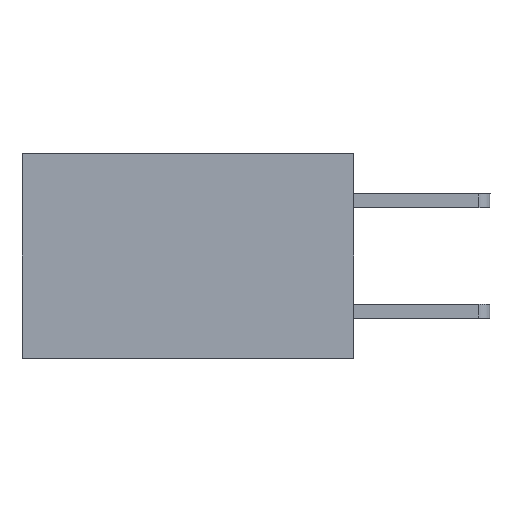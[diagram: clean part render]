
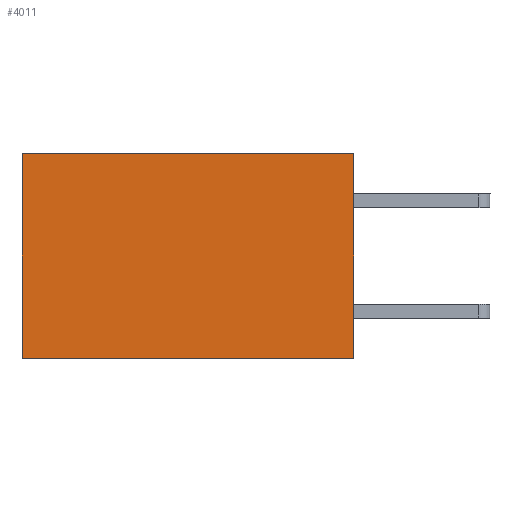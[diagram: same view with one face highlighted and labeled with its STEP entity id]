
A CAD part, left-side view. The second image highlights one B-rep face of the part: STEP entity #4011.
In plain terms, the highlighted planar face has unit normal (-1, 0, 0).
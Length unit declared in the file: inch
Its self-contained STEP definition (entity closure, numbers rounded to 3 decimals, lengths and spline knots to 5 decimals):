
#137 = VERTEX_POINT ( 'NONE', #3041 ) ;
#629 = VERTEX_POINT ( 'NONE', #8967 ) ;
#1329 = CARTESIAN_POINT ( 'NONE',  ( 0.2875, 0., -0.37 ) ) ;
#1948 = DIRECTION ( 'NONE',  ( 0., 0., -1. ) ) ;
#2176 = VECTOR ( 'NONE', #7032, 39.37008 ) ;
#2194 = ORIENTED_EDGE ( 'NONE', *, *, #3155, .T. ) ;
#2203 = CARTESIAN_POINT ( 'NONE',  ( 0.2875, 0., 0. ) ) ;
#2215 = EDGE_CURVE ( 'NONE', #8584, #6229, #4399, .T. ) ;
#2803 = LINE ( 'NONE', #6075, #2176 ) ;
#3041 = CARTESIAN_POINT ( 'NONE',  ( 0.2875, 0.6, -0.37 ) ) ;
#3075 = LINE ( 'NONE', #1329, #7894 ) ;
#3109 = VECTOR ( 'NONE', #10607, 39.37008 ) ;
#3155 = EDGE_CURVE ( 'NONE', #629, #137, #8492, .T. ) ;
#3424 = FACE_OUTER_BOUND ( 'NONE', #11330, .T. ) ;
#3886 = ORIENTED_EDGE ( 'NONE', *, *, #2215, .F. ) ;
#3895 = DIRECTION ( 'NONE',  ( 0., 0., -1. ) ) ;
#3902 = DIRECTION ( 'NONE',  ( 1., 0., 0. ) ) ;
#3924 = PLANE ( 'NONE',  #5825 ) ;
#4011 = ADVANCED_FACE ( 'NONE', ( #3424 ), #3924, .F. ) ;
#4056 = CARTESIAN_POINT ( 'NONE',  ( 0.2875, 0., 0. ) ) ;
#4399 = LINE ( 'NONE', #2203, #9074 ) ;
#4929 = CARTESIAN_POINT ( 'NONE',  ( 0.2875, 0., -0.37 ) ) ;
#5618 = ORIENTED_EDGE ( 'NONE', *, *, #7978, .T. ) ;
#5825 = AXIS2_PLACEMENT_3D ( 'NONE', #4056, #3902, #3895 ) ;
#6075 = CARTESIAN_POINT ( 'NONE',  ( 0.2875, 0., 0. ) ) ;
#6229 = VERTEX_POINT ( 'NONE', #4929 ) ;
#7032 = DIRECTION ( 'NONE',  ( 0., 1., 0. ) ) ;
#7894 = VECTOR ( 'NONE', #9043, 39.37008 ) ;
#7978 = EDGE_CURVE ( 'NONE', #8584, #629, #2803, .T. ) ;
#8492 = LINE ( 'NONE', #10238, #3109 ) ;
#8584 = VERTEX_POINT ( 'NONE', #11512 ) ;
#8967 = CARTESIAN_POINT ( 'NONE',  ( 0.2875, 0.6, 0. ) ) ;
#9043 = DIRECTION ( 'NONE',  ( 0., 1., 0. ) ) ;
#9074 = VECTOR ( 'NONE', #1948, 39.37008 ) ;
#9308 = ORIENTED_EDGE ( 'NONE', *, *, #10264, .F. ) ;
#10238 = CARTESIAN_POINT ( 'NONE',  ( 0.2875, 0.6, 0. ) ) ;
#10264 = EDGE_CURVE ( 'NONE', #6229, #137, #3075, .T. ) ;
#10607 = DIRECTION ( 'NONE',  ( 0., 0., -1. ) ) ;
#11330 = EDGE_LOOP ( 'NONE', ( #2194, #9308, #3886, #5618 ) ) ;
#11512 = CARTESIAN_POINT ( 'NONE',  ( 0.2875, 0., 0. ) ) ;
